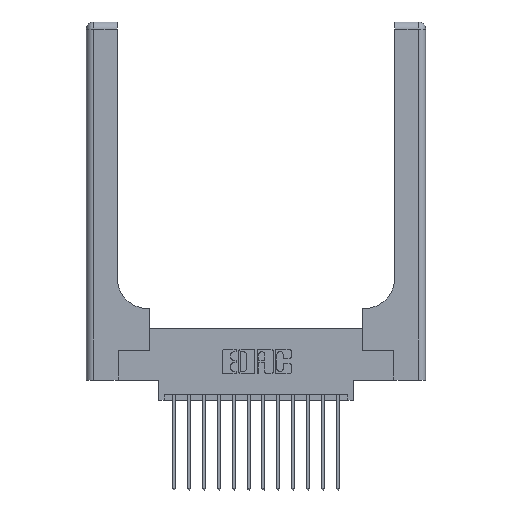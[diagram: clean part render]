
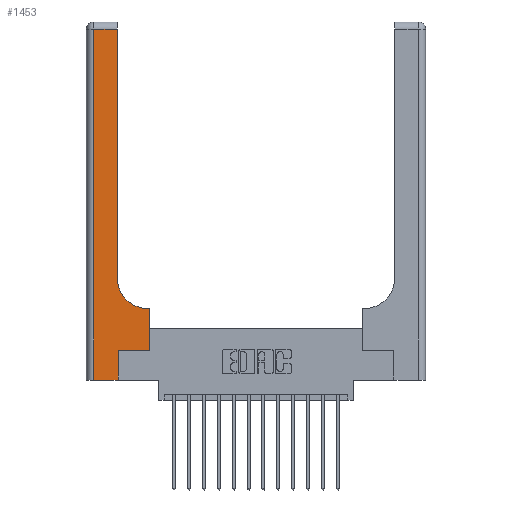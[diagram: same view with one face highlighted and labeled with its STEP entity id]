
A CAD part, top view. The second image highlights one B-rep face of the part: STEP entity #1453.
In plain terms, the highlighted planar face has unit normal (0, 0, 1).
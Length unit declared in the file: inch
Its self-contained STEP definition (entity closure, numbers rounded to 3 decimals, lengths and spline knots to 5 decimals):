
#148 = CARTESIAN_POINT ( 'NONE',  ( 0., 2.94, 0.37 ) ) ;
#215 = EDGE_CURVE ( 'NONE', #3299, #14620, #2899, .T. ) ;
#445 = LINE ( 'NONE', #5894, #9449 ) ;
#1210 = ORIENTED_EDGE ( 'NONE', *, *, #9240, .T. ) ;
#1328 = ORIENTED_EDGE ( 'NONE', *, *, #8059, .T. ) ;
#1403 = VERTEX_POINT ( 'NONE', #14867 ) ;
#1412 = VERTEX_POINT ( 'NONE', #8020 ) ;
#1453 = ADVANCED_FACE ( 'NONE', ( #6594 ), #7931, .F. ) ;
#1649 = DIRECTION ( 'NONE',  ( 0., 1., 0. ) ) ;
#1659 = VECTOR ( 'NONE', #12143, 39.37008 ) ;
#2051 = VECTOR ( 'NONE', #16579, 39.37008 ) ;
#2115 = ORIENTED_EDGE ( 'NONE', *, *, #215, .T. ) ;
#2586 = ORIENTED_EDGE ( 'NONE', *, *, #7745, .T. ) ;
#2730 = CIRCLE ( 'NONE', #9275, 0.25 ) ;
#2899 = LINE ( 'NONE', #5666, #4062 ) ;
#2916 = LINE ( 'NONE', #16392, #10440 ) ;
#3299 = VERTEX_POINT ( 'NONE', #13989 ) ;
#3674 = VERTEX_POINT ( 'NONE', #16657 ) ;
#4062 = VECTOR ( 'NONE', #1649, 39.37008 ) ;
#4632 = CARTESIAN_POINT ( 'NONE',  ( 0.06, 3., 0.37 ) ) ;
#5290 = EDGE_CURVE ( 'NONE', #11082, #16599, #2730, .T. ) ;
#5373 = EDGE_LOOP ( 'NONE', ( #2586, #8216, #16171, #9161, #2115, #1328, #15697, #1210, #13638 ) ) ;
#5428 = LINE ( 'NONE', #14870, #13412 ) ;
#5666 = CARTESIAN_POINT ( 'NONE',  ( 0.265, 0., 0.37 ) ) ;
#5694 = LINE ( 'NONE', #4632, #2051 ) ;
#5894 = CARTESIAN_POINT ( 'NONE',  ( 0.26, 3., 0.37 ) ) ;
#6097 = VECTOR ( 'NONE', #16577, 39.37008 ) ;
#6330 = DIRECTION ( 'NONE',  ( -1., 0., 0. ) ) ;
#6455 = LINE ( 'NONE', #9298, #1659 ) ;
#6594 = FACE_OUTER_BOUND ( 'NONE', #5373, .T. ) ;
#6822 = DIRECTION ( 'NONE',  ( 1., 0., 0. ) ) ;
#7678 = VERTEX_POINT ( 'NONE', #12473 ) ;
#7745 = EDGE_CURVE ( 'NONE', #16599, #1403, #445, .T. ) ;
#7931 = PLANE ( 'NONE',  #15221 ) ;
#8020 = CARTESIAN_POINT ( 'NONE',  ( 0.06, 2.94, 0.37 ) ) ;
#8059 = EDGE_CURVE ( 'NONE', #14620, #7678, #5428, .T. ) ;
#8130 = EDGE_CURVE ( 'NONE', #1412, #8917, #5694, .T. ) ;
#8216 = ORIENTED_EDGE ( 'NONE', *, *, #13545, .T. ) ;
#8467 = DIRECTION ( 'NONE',  ( 0., 1., 0. ) ) ;
#8917 = VERTEX_POINT ( 'NONE', #13410 ) ;
#9161 = ORIENTED_EDGE ( 'NONE', *, *, #15356, .T. ) ;
#9240 = EDGE_CURVE ( 'NONE', #3674, #11082, #17398, .T. ) ;
#9275 = AXIS2_PLACEMENT_3D ( 'NONE', #15183, #16638, #6822 ) ;
#9298 = CARTESIAN_POINT ( 'NONE',  ( 0.528, 0.25, 0.37 ) ) ;
#9348 = DIRECTION ( 'NONE',  ( 1., 0., 0. ) ) ;
#9449 = VECTOR ( 'NONE', #8467, 39.37008 ) ;
#9514 = DIRECTION ( 'NONE',  ( 0., 0., -1. ) ) ;
#9660 = VECTOR ( 'NONE', #6330, 39.37008 ) ;
#10440 = VECTOR ( 'NONE', #12535, 39.37008 ) ;
#10599 = CARTESIAN_POINT ( 'NONE',  ( 0.26, 0.6, 0.37 ) ) ;
#10609 = EDGE_CURVE ( 'NONE', #7678, #3674, #6455, .T. ) ;
#11082 = VERTEX_POINT ( 'NONE', #16513 ) ;
#12143 = DIRECTION ( 'NONE',  ( 0., 1., 0. ) ) ;
#12473 = CARTESIAN_POINT ( 'NONE',  ( 0.528, 0.25, 0.37 ) ) ;
#12535 = DIRECTION ( 'NONE',  ( 1., 0., 0. ) ) ;
#13410 = CARTESIAN_POINT ( 'NONE',  ( 0.06, 0., 0.37 ) ) ;
#13412 = VECTOR ( 'NONE', #9348, 39.37008 ) ;
#13545 = EDGE_CURVE ( 'NONE', #1403, #1412, #13711, .T. ) ;
#13623 = CARTESIAN_POINT ( 'NONE',  ( 0., 3., 0.37 ) ) ;
#13638 = ORIENTED_EDGE ( 'NONE', *, *, #5290, .T. ) ;
#13711 = LINE ( 'NONE', #148, #6097 ) ;
#13989 = CARTESIAN_POINT ( 'NONE',  ( 0.265, 0., 0.37 ) ) ;
#14620 = VERTEX_POINT ( 'NONE', #15797 ) ;
#14867 = CARTESIAN_POINT ( 'NONE',  ( 0.26, 2.94, 0.37 ) ) ;
#14870 = CARTESIAN_POINT ( 'NONE',  ( 0.265, 0.25, 0.37 ) ) ;
#15183 = CARTESIAN_POINT ( 'NONE',  ( 0.51, 0.85, 0.37 ) ) ;
#15221 = AXIS2_PLACEMENT_3D ( 'NONE', #13623, #9514, #17478 ) ;
#15356 = EDGE_CURVE ( 'NONE', #8917, #3299, #2916, .T. ) ;
#15403 = CARTESIAN_POINT ( 'NONE',  ( 0.26, 0.85, 0.37 ) ) ;
#15697 = ORIENTED_EDGE ( 'NONE', *, *, #10609, .T. ) ;
#15797 = CARTESIAN_POINT ( 'NONE',  ( 0.265, 0.25, 0.37 ) ) ;
#16171 = ORIENTED_EDGE ( 'NONE', *, *, #8130, .T. ) ;
#16392 = CARTESIAN_POINT ( 'NONE',  ( 0., 0., 0.37 ) ) ;
#16513 = CARTESIAN_POINT ( 'NONE',  ( 0.51, 0.6, 0.37 ) ) ;
#16577 = DIRECTION ( 'NONE',  ( -1., 0., 0. ) ) ;
#16579 = DIRECTION ( 'NONE',  ( 0., -1., 0. ) ) ;
#16599 = VERTEX_POINT ( 'NONE', #15403 ) ;
#16638 = DIRECTION ( 'NONE',  ( 0., 0., -1. ) ) ;
#16657 = CARTESIAN_POINT ( 'NONE',  ( 0.528, 0.6, 0.37 ) ) ;
#17398 = LINE ( 'NONE', #10599, #9660 ) ;
#17478 = DIRECTION ( 'NONE',  ( -1., 0., 0. ) ) ;
